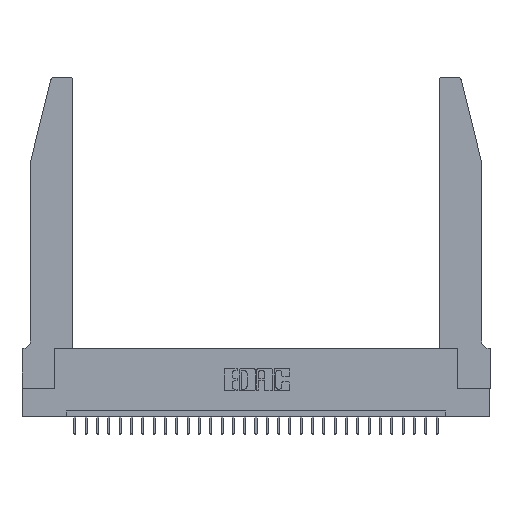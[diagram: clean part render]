
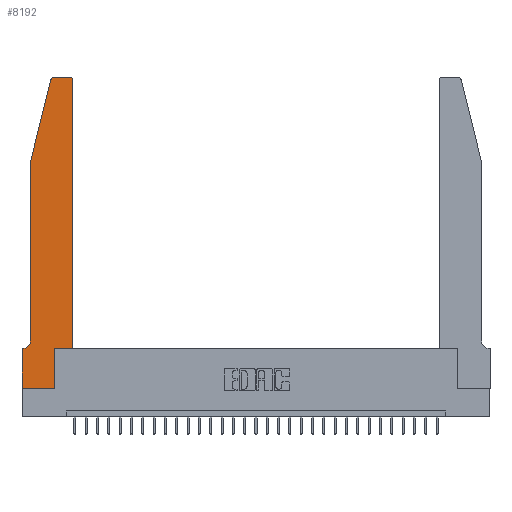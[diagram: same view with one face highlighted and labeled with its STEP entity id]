
A CAD part, top view. The second image highlights one B-rep face of the part: STEP entity #8192.
In plain terms, the highlighted planar face has unit normal (0, 0, 1).
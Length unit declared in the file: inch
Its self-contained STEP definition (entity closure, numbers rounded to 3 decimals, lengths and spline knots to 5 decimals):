
#72 = LINE ( 'NONE', #22952, #20910 ) ;
#271 = VECTOR ( 'NONE', #25245, 39.37008 ) ;
#627 = LINE ( 'NONE', #13454, #271 ) ;
#821 = VECTOR ( 'NONE', #1979, 39.37008 ) ;
#1197 = CARTESIAN_POINT ( 'NONE',  ( 0.0755, 0.42, 0.37 ) ) ;
#1303 = CARTESIAN_POINT ( 'NONE',  ( 0., 0., 0.37 ) ) ;
#1762 = CARTESIAN_POINT ( 'NONE',  ( 0.4205, 2.72, 0.37 ) ) ;
#1966 = ORIENTED_EDGE ( 'NONE', *, *, #2101, .T. ) ;
#1979 = DIRECTION ( 'NONE',  ( 1., 0., 0. ) ) ;
#2044 = EDGE_CURVE ( 'NONE', #9507, #18650, #5537, .T. ) ;
#2101 = EDGE_CURVE ( 'NONE', #5993, #22456, #30121, .T. ) ;
#2284 = VECTOR ( 'NONE', #19819, 39.37008 ) ;
#2554 = ORIENTED_EDGE ( 'NONE', *, *, #10926, .T. ) ;
#2712 = CARTESIAN_POINT ( 'NONE',  ( 0.0755, 0.35, 0.37 ) ) ;
#3306 = CARTESIAN_POINT ( 'NONE',  ( 0.2865, 0.35, 0.37 ) ) ;
#4260 = DIRECTION ( 'NONE',  ( 0., 0., -1. ) ) ;
#4386 = CARTESIAN_POINT ( 'NONE',  ( 0.0755, 2., 0.37 ) ) ;
#4831 = AXIS2_PLACEMENT_3D ( 'NONE', #1762, #20797, #18950 ) ;
#5537 = CIRCLE ( 'NONE', #4831, 0.03 ) ;
#5719 = CARTESIAN_POINT ( 'NONE',  ( 0.0055, 0.35, 0.37 ) ) ;
#5905 = DIRECTION ( 'NONE',  ( -1., 0., 0. ) ) ;
#5959 = FACE_OUTER_BOUND ( 'NONE', #13144, .T. ) ;
#5978 = VERTEX_POINT ( 'NONE', #30677 ) ;
#5993 = VERTEX_POINT ( 'NONE', #5719 ) ;
#6140 = VERTEX_POINT ( 'NONE', #16382 ) ;
#6374 = EDGE_CURVE ( 'NONE', #18650, #29747, #72, .T. ) ;
#6438 = LINE ( 'NONE', #8973, #821 ) ;
#7908 = EDGE_CURVE ( 'NONE', #6140, #9507, #8454, .T. ) ;
#8192 = ADVANCED_FACE ( 'NONE', ( #5959 ), #20299, .T. ) ;
#8395 = CARTESIAN_POINT ( 'NONE',  ( 0., 0., 0.37 ) ) ;
#8454 = LINE ( 'NONE', #30619, #24825 ) ;
#8463 = ORIENTED_EDGE ( 'NONE', *, *, #13951, .T. ) ;
#8973 = CARTESIAN_POINT ( 'NONE',  ( 0.4505, 0.35, 0.37 ) ) ;
#9427 = DIRECTION ( 'NONE',  ( 0., 0., 1. ) ) ;
#9507 = VERTEX_POINT ( 'NONE', #13706 ) ;
#9608 = LINE ( 'NONE', #8395, #13328 ) ;
#9668 = EDGE_CURVE ( 'NONE', #22456, #5978, #9608, .T. ) ;
#9736 = CARTESIAN_POINT ( 'NONE',  ( 0.0755, 2., 0.37 ) ) ;
#10197 = ORIENTED_EDGE ( 'NONE', *, *, #2044, .T. ) ;
#10391 = CARTESIAN_POINT ( 'NONE',  ( 0.4205, 2.75, 0.37 ) ) ;
#10916 = LINE ( 'NONE', #4386, #22750 ) ;
#10926 = EDGE_CURVE ( 'NONE', #29747, #26585, #28847, .T. ) ;
#10928 = DIRECTION ( 'NONE',  ( 1., 0., 0. ) ) ;
#11201 = ORIENTED_EDGE ( 'NONE', *, *, #6374, .T. ) ;
#11352 = DIRECTION ( 'NONE',  ( -1., 0., 0. ) ) ;
#12799 = CARTESIAN_POINT ( 'NONE',  ( 0.284, 2.75, 0.37 ) ) ;
#13034 = VECTOR ( 'NONE', #10928, 39.37008 ) ;
#13144 = EDGE_LOOP ( 'NONE', ( #11201, #2554, #25407, #19396, #13764, #1966, #25636, #29319, #8463, #27813, #15465, #10197 ) ) ;
#13328 = VECTOR ( 'NONE', #27301, 39.37008 ) ;
#13454 = CARTESIAN_POINT ( 'NONE',  ( 0.0755, 2., 0.37 ) ) ;
#13706 = CARTESIAN_POINT ( 'NONE',  ( 0.4505, 2.72, 0.37 ) ) ;
#13764 = ORIENTED_EDGE ( 'NONE', *, *, #29976, .T. ) ;
#13951 = EDGE_CURVE ( 'NONE', #21755, #24058, #23044, .T. ) ;
#14507 = DIRECTION ( 'NONE',  ( 1., 0., 0. ) ) ;
#15272 = AXIS2_PLACEMENT_3D ( 'NONE', #23253, #4260, #11352 ) ;
#15465 = ORIENTED_EDGE ( 'NONE', *, *, #7908, .T. ) ;
#15905 = VERTEX_POINT ( 'NONE', #1197 ) ;
#15920 = EDGE_CURVE ( 'NONE', #5978, #21755, #19340, .T. ) ;
#16048 = DIRECTION ( 'NONE',  ( 0., 1., 0. ) ) ;
#16382 = CARTESIAN_POINT ( 'NONE',  ( 0.4505, 0.35, 0.37 ) ) ;
#16504 = DIRECTION ( 'NONE',  ( 1., 0., 0. ) ) ;
#18102 = CARTESIAN_POINT ( 'NONE',  ( 0., 0.35, 0.37 ) ) ;
#18650 = VERTEX_POINT ( 'NONE', #10391 ) ;
#18950 = DIRECTION ( 'NONE',  ( 1., 0., 0. ) ) ;
#19340 = LINE ( 'NONE', #1303, #13034 ) ;
#19396 = ORIENTED_EDGE ( 'NONE', *, *, #24971, .T. ) ;
#19819 = DIRECTION ( 'NONE',  ( 0., 1., 0. ) ) ;
#20299 = PLANE ( 'NONE',  #20543 ) ;
#20529 = CIRCLE ( 'NONE', #15272, 0.07 ) ;
#20543 = AXIS2_PLACEMENT_3D ( 'NONE', #25909, #30764, #16504 ) ;
#20797 = DIRECTION ( 'NONE',  ( 0., 0., 1. ) ) ;
#20910 = VECTOR ( 'NONE', #30265, 39.37008 ) ;
#21755 = VERTEX_POINT ( 'NONE', #23244 ) ;
#22456 = VERTEX_POINT ( 'NONE', #18102 ) ;
#22477 = EDGE_CURVE ( 'NONE', #26585, #27922, #627, .T. ) ;
#22750 = VECTOR ( 'NONE', #23173, 39.37008 ) ;
#22952 = CARTESIAN_POINT ( 'NONE',  ( 0.2605, 2.75, 0.37 ) ) ;
#23044 = LINE ( 'NONE', #3306, #2284 ) ;
#23173 = DIRECTION ( 'NONE',  ( 0., -1., 0. ) ) ;
#23244 = CARTESIAN_POINT ( 'NONE',  ( 0.2865, 0., 0.37 ) ) ;
#23253 = CARTESIAN_POINT ( 'NONE',  ( 0.0055, 0.42, 0.37 ) ) ;
#24058 = VERTEX_POINT ( 'NONE', #27616 ) ;
#24290 = CARTESIAN_POINT ( 'NONE',  ( 0.25487, 2.72718, 0.37 ) ) ;
#24825 = VECTOR ( 'NONE', #16048, 39.37008 ) ;
#24957 = EDGE_CURVE ( 'NONE', #24058, #6140, #6438, .T. ) ;
#24971 = EDGE_CURVE ( 'NONE', #27922, #15905, #10916, .T. ) ;
#25245 = DIRECTION ( 'NONE',  ( -0.239, -0.971, 0. ) ) ;
#25407 = ORIENTED_EDGE ( 'NONE', *, *, #22477, .T. ) ;
#25636 = ORIENTED_EDGE ( 'NONE', *, *, #9668, .T. ) ;
#25909 = CARTESIAN_POINT ( 'NONE',  ( 0., 0.35, 0.37 ) ) ;
#26585 = VERTEX_POINT ( 'NONE', #24290 ) ;
#27301 = DIRECTION ( 'NONE',  ( 0., -1., 0. ) ) ;
#27616 = CARTESIAN_POINT ( 'NONE',  ( 0.2865, 0.35, 0.37 ) ) ;
#27813 = ORIENTED_EDGE ( 'NONE', *, *, #24957, .T. ) ;
#27851 = VECTOR ( 'NONE', #5905, 39.37008 ) ;
#27922 = VERTEX_POINT ( 'NONE', #9736 ) ;
#28216 = CARTESIAN_POINT ( 'NONE',  ( 0.284, 2.72, 0.37 ) ) ;
#28847 = CIRCLE ( 'NONE', #29588, 0.03 ) ;
#29319 = ORIENTED_EDGE ( 'NONE', *, *, #15920, .T. ) ;
#29588 = AXIS2_PLACEMENT_3D ( 'NONE', #28216, #9427, #14507 ) ;
#29747 = VERTEX_POINT ( 'NONE', #12799 ) ;
#29976 = EDGE_CURVE ( 'NONE', #15905, #5993, #20529, .T. ) ;
#30121 = LINE ( 'NONE', #2712, #27851 ) ;
#30265 = DIRECTION ( 'NONE',  ( -1., 0., 0. ) ) ;
#30619 = CARTESIAN_POINT ( 'NONE',  ( 0.4505, 0.35, 0.37 ) ) ;
#30677 = CARTESIAN_POINT ( 'NONE',  ( 0., 0., 0.37 ) ) ;
#30764 = DIRECTION ( 'NONE',  ( 0., 0., 1. ) ) ;
